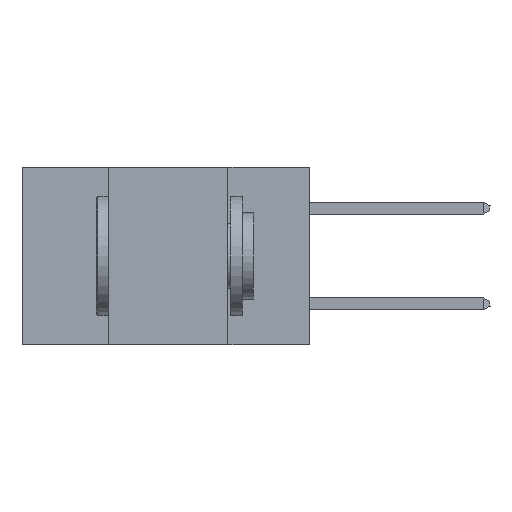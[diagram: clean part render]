
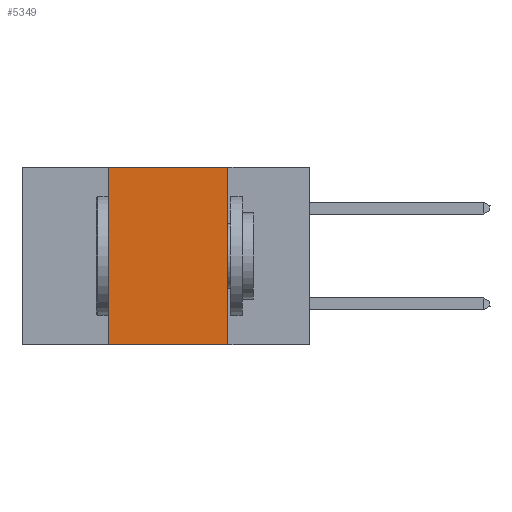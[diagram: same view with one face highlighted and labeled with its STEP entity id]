
A CAD part, left-side view. The second image highlights one B-rep face of the part: STEP entity #5349.
In plain terms, the highlighted planar face has unit normal (-1, 0, 0).
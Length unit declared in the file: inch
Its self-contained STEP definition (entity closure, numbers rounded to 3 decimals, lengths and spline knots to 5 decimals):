
#454 = DIRECTION ( 'NONE',  ( 0., 0., -1. ) ) ;
#1729 = EDGE_CURVE ( 'NONE', #3779, #12083, #4755, .T. ) ;
#1736 = CARTESIAN_POINT ( 'NONE',  ( 0., 0.42, 0. ) ) ;
#1989 = ORIENTED_EDGE ( 'NONE', *, *, #8801, .F. ) ;
#2379 = CARTESIAN_POINT ( 'NONE',  ( 0., 0.42, 0. ) ) ;
#2860 = LINE ( 'NONE', #1736, #9450 ) ;
#3779 = VERTEX_POINT ( 'NONE', #10465 ) ;
#4011 = AXIS2_PLACEMENT_3D ( 'NONE', #16967, #14159, #7280 ) ;
#4755 = LINE ( 'NONE', #14830, #17880 ) ;
#4946 = ORIENTED_EDGE ( 'NONE', *, *, #7013, .F. ) ;
#5065 = VERTEX_POINT ( 'NONE', #13604 ) ;
#5123 = CARTESIAN_POINT ( 'NONE',  ( 0., 0.17, 0. ) ) ;
#5349 = ADVANCED_FACE ( 'NONE', ( #7267 ), #15678, .F. ) ;
#5363 = EDGE_CURVE ( 'NONE', #3779, #7868, #2860, .T. ) ;
#5390 = CARTESIAN_POINT ( 'NONE',  ( 0., 0.6, 0. ) ) ;
#6503 = VECTOR ( 'NONE', #15205, 39.37008 ) ;
#6937 = CARTESIAN_POINT ( 'NONE',  ( 0., 0.17, -0.37 ) ) ;
#7013 = EDGE_CURVE ( 'NONE', #5065, #12083, #13574, .T. ) ;
#7267 = FACE_OUTER_BOUND ( 'NONE', #13907, .T. ) ;
#7280 = DIRECTION ( 'NONE',  ( 0., 0., -1. ) ) ;
#7868 = VERTEX_POINT ( 'NONE', #2379 ) ;
#7890 = ORIENTED_EDGE ( 'NONE', *, *, #1729, .T. ) ;
#8052 = VECTOR ( 'NONE', #454, 39.37008 ) ;
#8801 = EDGE_CURVE ( 'NONE', #7868, #5065, #17668, .T. ) ;
#9187 = DIRECTION ( 'NONE',  ( 0., -1., 0. ) ) ;
#9450 = VECTOR ( 'NONE', #9962, 39.37008 ) ;
#9962 = DIRECTION ( 'NONE',  ( 0., 0., 1. ) ) ;
#10321 = ORIENTED_EDGE ( 'NONE', *, *, #5363, .F. ) ;
#10465 = CARTESIAN_POINT ( 'NONE',  ( 0., 0.42, -0.37 ) ) ;
#12083 = VERTEX_POINT ( 'NONE', #6937 ) ;
#13574 = LINE ( 'NONE', #5123, #8052 ) ;
#13604 = CARTESIAN_POINT ( 'NONE',  ( 0., 0.17, 0. ) ) ;
#13907 = EDGE_LOOP ( 'NONE', ( #4946, #1989, #10321, #7890 ) ) ;
#14159 = DIRECTION ( 'NONE',  ( 1., 0., 0. ) ) ;
#14830 = CARTESIAN_POINT ( 'NONE',  ( 0., 0.6, -0.37 ) ) ;
#15205 = DIRECTION ( 'NONE',  ( 0., -1., 0. ) ) ;
#15678 = PLANE ( 'NONE',  #4011 ) ;
#16967 = CARTESIAN_POINT ( 'NONE',  ( 0., 0.6, 0. ) ) ;
#17668 = LINE ( 'NONE', #5390, #6503 ) ;
#17880 = VECTOR ( 'NONE', #9187, 39.37008 ) ;
